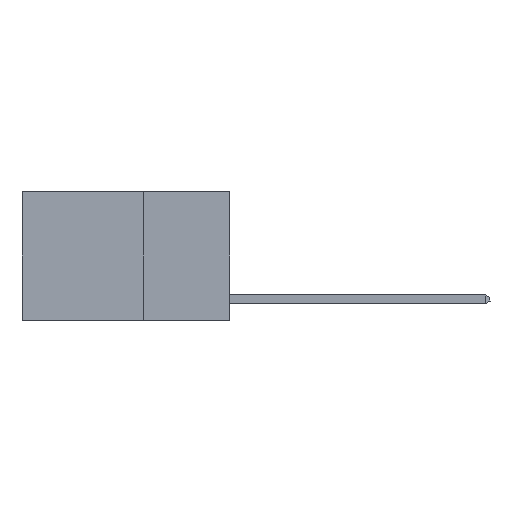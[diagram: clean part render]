
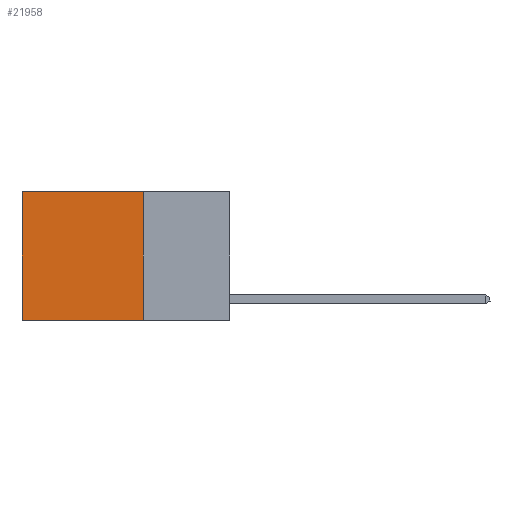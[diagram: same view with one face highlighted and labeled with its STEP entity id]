
A CAD part, left-side view. The second image highlights one B-rep face of the part: STEP entity #21958.
In plain terms, the highlighted planar face has unit normal (-1, 0, 0).
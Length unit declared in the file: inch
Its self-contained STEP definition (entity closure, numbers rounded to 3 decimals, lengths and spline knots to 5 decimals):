
#634 = DIRECTION ( 'NONE',  ( 1., 0., 0. ) ) ;
#1816 = VERTEX_POINT ( 'NONE', #17415 ) ;
#2418 = CARTESIAN_POINT ( 'NONE',  ( 0.2625, 0.6, -0.37 ) ) ;
#2543 = CARTESIAN_POINT ( 'NONE',  ( 0.2625, 0.25, 0. ) ) ;
#4647 = VERTEX_POINT ( 'NONE', #6172 ) ;
#6172 = CARTESIAN_POINT ( 'NONE',  ( 0.2625, 0.25, -0.37 ) ) ;
#6590 = VERTEX_POINT ( 'NONE', #8649 ) ;
#7977 = ORIENTED_EDGE ( 'NONE', *, *, #19082, .F. ) ;
#8649 = CARTESIAN_POINT ( 'NONE',  ( 0.2625, 0.25, 0. ) ) ;
#10370 = VECTOR ( 'NONE', #16470, 39.37008 ) ;
#10697 = DIRECTION ( 'NONE',  ( 0., 0., -1. ) ) ;
#11885 = VECTOR ( 'NONE', #22720, 39.37008 ) ;
#12392 = PLANE ( 'NONE',  #18151 ) ;
#12666 = LINE ( 'NONE', #15151, #14286 ) ;
#14213 = VERTEX_POINT ( 'NONE', #2418 ) ;
#14286 = VECTOR ( 'NONE', #21515, 39.37008 ) ;
#14363 = EDGE_CURVE ( 'NONE', #6590, #1816, #12666, .T. ) ;
#15151 = CARTESIAN_POINT ( 'NONE',  ( 0.2625, 0.25, 0. ) ) ;
#15610 = EDGE_CURVE ( 'NONE', #1816, #14213, #21544, .T. ) ;
#16111 = CARTESIAN_POINT ( 'NONE',  ( 0.2625, 0.25, -0.37 ) ) ;
#16132 = FACE_OUTER_BOUND ( 'NONE', #23708, .T. ) ;
#16181 = LINE ( 'NONE', #20910, #25877 ) ;
#16470 = DIRECTION ( 'NONE',  ( 0., 1., 0. ) ) ;
#17415 = CARTESIAN_POINT ( 'NONE',  ( 0.2625, 0.6, 0. ) ) ;
#18151 = AXIS2_PLACEMENT_3D ( 'NONE', #2543, #634, #10697 ) ;
#18161 = LINE ( 'NONE', #16111, #10370 ) ;
#19011 = CARTESIAN_POINT ( 'NONE',  ( 0.2625, 0.6, 0. ) ) ;
#19082 = EDGE_CURVE ( 'NONE', #4647, #14213, #18161, .T. ) ;
#19760 = EDGE_CURVE ( 'NONE', #6590, #4647, #16181, .T. ) ;
#20383 = DIRECTION ( 'NONE',  ( 0., 0., -1. ) ) ;
#20910 = CARTESIAN_POINT ( 'NONE',  ( 0.2625, 0.25, 0. ) ) ;
#21515 = DIRECTION ( 'NONE',  ( 0., 1., 0. ) ) ;
#21544 = LINE ( 'NONE', #19011, #11885 ) ;
#21939 = ORIENTED_EDGE ( 'NONE', *, *, #14363, .T. ) ;
#21958 = ADVANCED_FACE ( 'NONE', ( #16132 ), #12392, .F. ) ;
#22622 = ORIENTED_EDGE ( 'NONE', *, *, #19760, .F. ) ;
#22720 = DIRECTION ( 'NONE',  ( 0., 0., -1. ) ) ;
#23708 = EDGE_LOOP ( 'NONE', ( #25008, #7977, #22622, #21939 ) ) ;
#25008 = ORIENTED_EDGE ( 'NONE', *, *, #15610, .T. ) ;
#25877 = VECTOR ( 'NONE', #20383, 39.37008 ) ;
